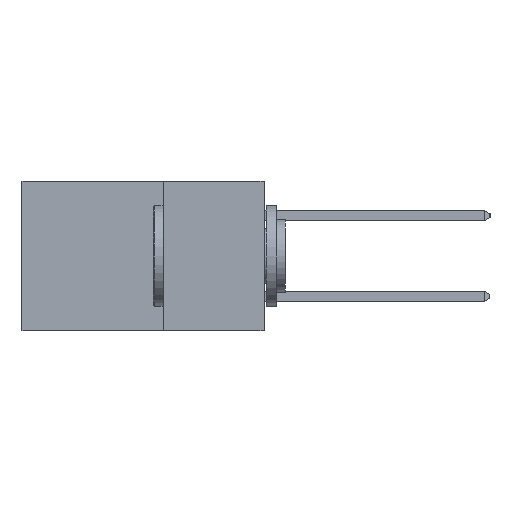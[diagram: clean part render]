
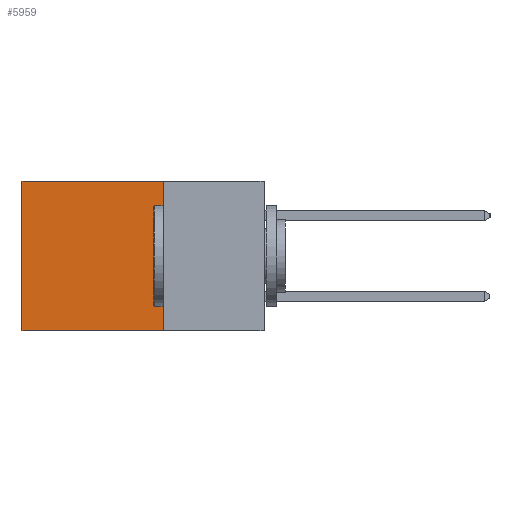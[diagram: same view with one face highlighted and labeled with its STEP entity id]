
A CAD part, left-side view. The second image highlights one B-rep face of the part: STEP entity #5959.
In plain terms, the highlighted planar face has unit normal (-1, 0, 0).
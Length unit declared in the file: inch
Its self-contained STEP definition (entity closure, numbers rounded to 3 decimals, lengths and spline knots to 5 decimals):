
#153 = VERTEX_POINT ( 'NONE', #19777 ) ;
#623 = DIRECTION ( 'NONE',  ( 0., 1., 0. ) ) ;
#652 = EDGE_CURVE ( 'NONE', #20601, #153, #15842, .T. ) ;
#669 = VERTEX_POINT ( 'NONE', #13385 ) ;
#2267 = CARTESIAN_POINT ( 'NONE',  ( 0.2615, 0.25, 0. ) ) ;
#2401 = LINE ( 'NONE', #5776, #18310 ) ;
#3390 = DIRECTION ( 'NONE',  ( 0., 0., -1. ) ) ;
#4143 = DIRECTION ( 'NONE',  ( 0., 1., 0. ) ) ;
#4146 = DIRECTION ( 'NONE',  ( 0., 0., -1. ) ) ;
#5776 = CARTESIAN_POINT ( 'NONE',  ( 0.2615, 0.25, -0.37 ) ) ;
#5794 = ORIENTED_EDGE ( 'NONE', *, *, #16704, .F. ) ;
#5959 = ADVANCED_FACE ( 'NONE', ( #12351 ), #18788, .F. ) ;
#7214 = EDGE_LOOP ( 'NONE', ( #16690, #14076, #5794, #20531 ) ) ;
#10457 = VECTOR ( 'NONE', #11638, 39.37008 ) ;
#11638 = DIRECTION ( 'NONE',  ( 0., 0., -1. ) ) ;
#12351 = FACE_OUTER_BOUND ( 'NONE', #7214, .T. ) ;
#13096 = VECTOR ( 'NONE', #623, 39.37008 ) ;
#13191 = CARTESIAN_POINT ( 'NONE',  ( 0.2615, 0.6, 0. ) ) ;
#13385 = CARTESIAN_POINT ( 'NONE',  ( 0.2615, 0.25, -0.37 ) ) ;
#14076 = ORIENTED_EDGE ( 'NONE', *, *, #16921, .F. ) ;
#14245 = AXIS2_PLACEMENT_3D ( 'NONE', #17024, #15417, #4146 ) ;
#14483 = CARTESIAN_POINT ( 'NONE',  ( 0.2615, 0.6, -0.37 ) ) ;
#15417 = DIRECTION ( 'NONE',  ( 1., 0., 0. ) ) ;
#15842 = LINE ( 'NONE', #14483, #10457 ) ;
#15880 = VECTOR ( 'NONE', #3390, 39.37008 ) ;
#16690 = ORIENTED_EDGE ( 'NONE', *, *, #652, .T. ) ;
#16703 = LINE ( 'NONE', #20003, #15880 ) ;
#16704 = EDGE_CURVE ( 'NONE', #19121, #669, #16703, .T. ) ;
#16921 = EDGE_CURVE ( 'NONE', #669, #153, #2401, .T. ) ;
#17024 = CARTESIAN_POINT ( 'NONE',  ( 0.2615, 0.25, -0.37 ) ) ;
#17388 = EDGE_CURVE ( 'NONE', #19121, #20601, #17428, .T. ) ;
#17428 = LINE ( 'NONE', #2267, #13096 ) ;
#17561 = CARTESIAN_POINT ( 'NONE',  ( 0.2615, 0.25, 0. ) ) ;
#18310 = VECTOR ( 'NONE', #4143, 39.37008 ) ;
#18788 = PLANE ( 'NONE',  #14245 ) ;
#19121 = VERTEX_POINT ( 'NONE', #17561 ) ;
#19777 = CARTESIAN_POINT ( 'NONE',  ( 0.2615, 0.6, -0.37 ) ) ;
#20003 = CARTESIAN_POINT ( 'NONE',  ( 0.2615, 0.25, -0.37 ) ) ;
#20531 = ORIENTED_EDGE ( 'NONE', *, *, #17388, .T. ) ;
#20601 = VERTEX_POINT ( 'NONE', #13191 ) ;
